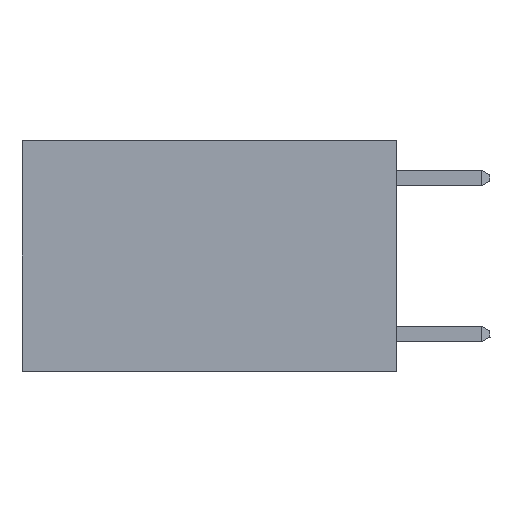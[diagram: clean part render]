
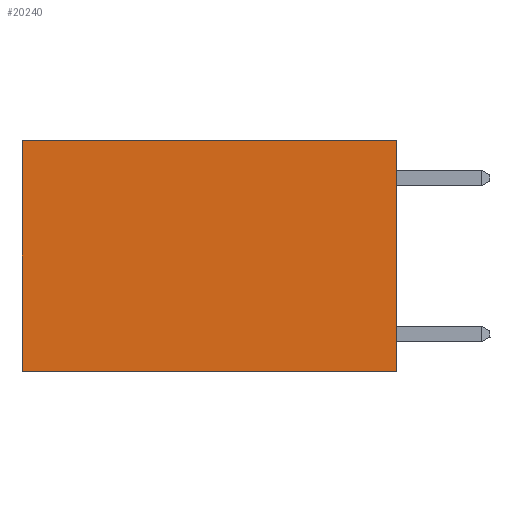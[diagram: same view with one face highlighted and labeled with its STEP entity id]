
A CAD part, left-side view. The second image highlights one B-rep face of the part: STEP entity #20240.
In plain terms, the highlighted planar face has unit normal (-1, 0, 0).
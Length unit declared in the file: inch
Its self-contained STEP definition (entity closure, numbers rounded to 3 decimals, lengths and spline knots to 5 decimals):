
#2325 = ORIENTED_EDGE ( 'NONE', *, *, #20169, .T. ) ;
#2343 = EDGE_CURVE ( 'NONE', #19597, #6032, #17825, .T. ) ;
#2671 = CARTESIAN_POINT ( 'NONE',  ( 0.2625, 0.6, 0. ) ) ;
#3594 = VECTOR ( 'NONE', #8831, 39.37008 ) ;
#3662 = LINE ( 'NONE', #18366, #3594 ) ;
#3675 = DIRECTION ( 'NONE',  ( 0., 1., 0. ) ) ;
#4494 = PLANE ( 'NONE',  #19618 ) ;
#6032 = VERTEX_POINT ( 'NONE', #6551 ) ;
#6162 = DIRECTION ( 'NONE',  ( 0., 0., -1. ) ) ;
#6551 = CARTESIAN_POINT ( 'NONE',  ( 0.2625, 0.6, -0.37 ) ) ;
#6867 = CARTESIAN_POINT ( 'NONE',  ( 0.2625, 0., -0.37 ) ) ;
#7917 = ORIENTED_EDGE ( 'NONE', *, *, #8556, .F. ) ;
#8556 = EDGE_CURVE ( 'NONE', #13577, #19251, #3662, .T. ) ;
#8831 = DIRECTION ( 'NONE',  ( 0., 0., -1. ) ) ;
#9314 = CARTESIAN_POINT ( 'NONE',  ( 0.2625, 0., 0. ) ) ;
#9468 = CARTESIAN_POINT ( 'NONE',  ( 0.2625, 0., 0. ) ) ;
#11592 = ORIENTED_EDGE ( 'NONE', *, *, #16073, .F. ) ;
#11736 = LINE ( 'NONE', #15120, #19956 ) ;
#12014 = ORIENTED_EDGE ( 'NONE', *, *, #2343, .T. ) ;
#12262 = EDGE_LOOP ( 'NONE', ( #12014, #11592, #7917, #2325 ) ) ;
#13577 = VERTEX_POINT ( 'NONE', #19879 ) ;
#14031 = VECTOR ( 'NONE', #18777, 39.37008 ) ;
#14238 = DIRECTION ( 'NONE',  ( 0., 0., -1. ) ) ;
#15120 = CARTESIAN_POINT ( 'NONE',  ( 0.2625, 0., -0.37 ) ) ;
#15847 = DIRECTION ( 'NONE',  ( 1., 0., 0. ) ) ;
#16073 = EDGE_CURVE ( 'NONE', #19251, #6032, #11736, .T. ) ;
#16670 = FACE_OUTER_BOUND ( 'NONE', #12262, .T. ) ;
#17269 = CARTESIAN_POINT ( 'NONE',  ( 0.2625, 0.6, 0. ) ) ;
#17581 = VECTOR ( 'NONE', #14238, 39.37008 ) ;
#17825 = LINE ( 'NONE', #17269, #17581 ) ;
#18177 = LINE ( 'NONE', #9314, #14031 ) ;
#18366 = CARTESIAN_POINT ( 'NONE',  ( 0.2625, 0., 0. ) ) ;
#18777 = DIRECTION ( 'NONE',  ( 0., 1., 0. ) ) ;
#19251 = VERTEX_POINT ( 'NONE', #6867 ) ;
#19597 = VERTEX_POINT ( 'NONE', #2671 ) ;
#19618 = AXIS2_PLACEMENT_3D ( 'NONE', #9468, #15847, #6162 ) ;
#19879 = CARTESIAN_POINT ( 'NONE',  ( 0.2625, 0., 0. ) ) ;
#19956 = VECTOR ( 'NONE', #3675, 39.37008 ) ;
#20169 = EDGE_CURVE ( 'NONE', #13577, #19597, #18177, .T. ) ;
#20240 = ADVANCED_FACE ( 'NONE', ( #16670 ), #4494, .F. ) ;
